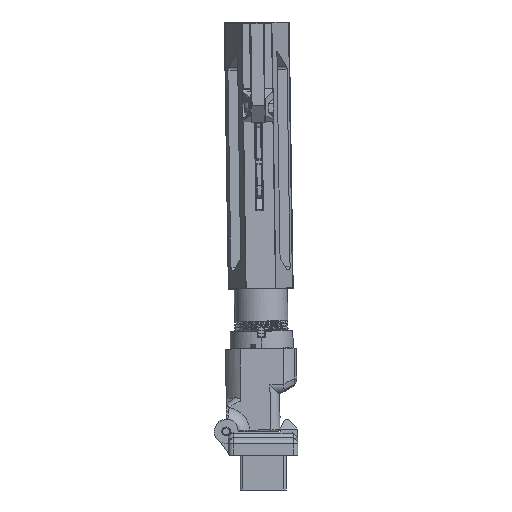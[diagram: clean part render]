
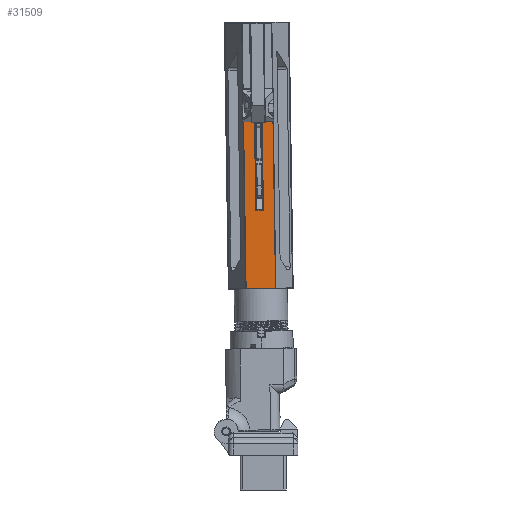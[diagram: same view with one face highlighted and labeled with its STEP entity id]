
A CAD part, front view. The second image highlights one B-rep face of the part: STEP entity #31509.
In plain terms, the highlighted planar face has unit normal (0.001, -1, 0).
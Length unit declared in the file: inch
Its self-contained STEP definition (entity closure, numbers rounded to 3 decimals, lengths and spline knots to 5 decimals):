
#1038 = DIRECTION ( 'NONE',  ( -1., 0., 0. ) ) ;
#1393 = EDGE_CURVE ( 'NONE', #83956, #16129, #110969, .T. ) ;
#1433 = LINE ( 'NONE', #73468, #92094 ) ;
#1583 = CARTESIAN_POINT ( 'NONE',  ( -0.20623, 2.27701, 0.60654 ) ) ;
#3004 = LINE ( 'NONE', #113807, #50618 ) ;
#4150 = CARTESIAN_POINT ( 'NONE',  ( 0.25882, 2.27701, 0.75605 ) ) ;
#4573 = EDGE_CURVE ( 'NONE', #48424, #16129, #3004, .T. ) ;
#5254 = VECTOR ( 'NONE', #115520, 39.37008 ) ;
#6679 = LINE ( 'NONE', #60556, #40078 ) ;
#7333 = VERTEX_POINT ( 'NONE', #119775 ) ;
#7878 = DIRECTION ( 'NONE',  ( -1., 0., 0. ) ) ;
#9898 = DIRECTION ( 'NONE',  ( 0., 0., 1. ) ) ;
#11533 = CARTESIAN_POINT ( 'NONE',  ( 0.25882, 2.27701, 4.21059 ) ) ;
#11699 = LINE ( 'NONE', #93976, #109061 ) ;
#12814 = VECTOR ( 'NONE', #1038, 39.37008 ) ;
#13151 = DIRECTION ( 'NONE',  ( 0., 0., -1. ) ) ;
#14095 = EDGE_CURVE ( 'NONE', #109037, #54313, #96042, .T. ) ;
#14333 = VERTEX_POINT ( 'NONE', #36059 ) ;
#14604 = EDGE_LOOP ( 'NONE', ( #80668, #86055, #26712, #99197, #62341, #112582, #38522, #43325, #58567, #66247, #104048, #114836 ) ) ;
#16129 = VERTEX_POINT ( 'NONE', #95921 ) ;
#17422 = VECTOR ( 'NONE', #95929, 39.37008 ) ;
#21709 = EDGE_CURVE ( 'NONE', #53142, #81474, #23504, .T. ) ;
#23504 = LINE ( 'NONE', #78538, #5254 ) ;
#26712 = ORIENTED_EDGE ( 'NONE', *, *, #64079, .T. ) ;
#28824 = VECTOR ( 'NONE', #64938, 39.37008 ) ;
#30843 = DIRECTION ( 'NONE',  ( 0., 0., -1. ) ) ;
#31509 = ADVANCED_FACE ( 'NONE', ( #77946 ), #68283, .T. ) ;
#32437 = LINE ( 'NONE', #69942, #37668 ) ;
#33949 = VECTOR ( 'NONE', #9898, 39.37008 ) ;
#34353 = CARTESIAN_POINT ( 'NONE',  ( 0.42972, 2.27701, 4.21059 ) ) ;
#36059 = CARTESIAN_POINT ( 'NONE',  ( 0.02853, 2.27701, 4.21414 ) ) ;
#37166 = AXIS2_PLACEMENT_3D ( 'NONE', #4150, #67688, #59822 ) ;
#37581 = VECTOR ( 'NONE', #13151, 39.37008 ) ;
#37668 = VECTOR ( 'NONE', #40341, 39.37008 ) ;
#38384 = DIRECTION ( 'NONE',  ( 0., 0., -1. ) ) ;
#38522 = ORIENTED_EDGE ( 'NONE', *, *, #71679, .T. ) ;
#40078 = VECTOR ( 'NONE', #7878, 39.37008 ) ;
#40341 = DIRECTION ( 'NONE',  ( -1., 0., 0. ) ) ;
#43325 = ORIENTED_EDGE ( 'NONE', *, *, #103541, .T. ) ;
#47232 = EDGE_CURVE ( 'NONE', #54313, #78135, #68656, .T. ) ;
#47954 = LINE ( 'NONE', #112142, #33949 ) ;
#48424 = VERTEX_POINT ( 'NONE', #67642 ) ;
#50618 = VECTOR ( 'NONE', #30843, 39.37008 ) ;
#53142 = VERTEX_POINT ( 'NONE', #85937 ) ;
#54313 = VERTEX_POINT ( 'NONE', #1583 ) ;
#58567 = ORIENTED_EDGE ( 'NONE', *, *, #105902, .T. ) ;
#59503 = CARTESIAN_POINT ( 'NONE',  ( -0.20623, 2.27701, 4.21059 ) ) ;
#59822 = DIRECTION ( 'NONE',  ( 0., 0., -1. ) ) ;
#60556 = CARTESIAN_POINT ( 'NONE',  ( 0.25882, 2.27701, 4.21414 ) ) ;
#61185 = VECTOR ( 'NONE', #65089, 39.37008 ) ;
#62341 = ORIENTED_EDGE ( 'NONE', *, *, #4573, .F. ) ;
#64079 = EDGE_CURVE ( 'NONE', #78135, #83956, #11699, .T. ) ;
#64938 = DIRECTION ( 'NONE',  ( -1., 0., 0. ) ) ;
#65089 = DIRECTION ( 'NONE',  ( -1., 0., 0. ) ) ;
#66247 = ORIENTED_EDGE ( 'NONE', *, *, #109834, .T. ) ;
#67489 = CARTESIAN_POINT ( 'NONE',  ( 0.42972, 2.27701, 0.60654 ) ) ;
#67642 = CARTESIAN_POINT ( 'NONE',  ( 0.25882, 2.27701, 4.21327 ) ) ;
#67688 = DIRECTION ( 'NONE',  ( 0., -1., 0. ) ) ;
#68283 = PLANE ( 'NONE',  #37166 ) ;
#68656 = LINE ( 'NONE', #77717, #17422 ) ;
#69942 = CARTESIAN_POINT ( 'NONE',  ( 0.25882, 2.27701, 2.2914 ) ) ;
#70063 = EDGE_CURVE ( 'NONE', #48424, #7333, #82619, .T. ) ;
#71679 = EDGE_CURVE ( 'NONE', #7333, #83482, #1433, .T. ) ;
#73468 = CARTESIAN_POINT ( 'NONE',  ( 0.19496, 2.27701, 0.75605 ) ) ;
#74956 = EDGE_CURVE ( 'NONE', #81474, #109037, #119142, .T. ) ;
#77717 = CARTESIAN_POINT ( 'NONE',  ( 0.42836, 2.27701, 0.60654 ) ) ;
#77946 = FACE_OUTER_BOUND ( 'NONE', #14604, .T. ) ;
#78135 = VERTEX_POINT ( 'NONE', #67489 ) ;
#78538 = CARTESIAN_POINT ( 'NONE',  ( -0.03533, 2.27701, 4.54102 ) ) ;
#80668 = ORIENTED_EDGE ( 'NONE', *, *, #14095, .T. ) ;
#81229 = CARTESIAN_POINT ( 'NONE',  ( -0.03533, 2.27701, 4.21059 ) ) ;
#81474 = VERTEX_POINT ( 'NONE', #81229 ) ;
#82619 = LINE ( 'NONE', #92325, #61185 ) ;
#83482 = VERTEX_POINT ( 'NONE', #107567 ) ;
#83933 = CARTESIAN_POINT ( 'NONE',  ( 0.25882, 2.27701, 4.21059 ) ) ;
#83956 = VERTEX_POINT ( 'NONE', #34353 ) ;
#85937 = CARTESIAN_POINT ( 'NONE',  ( -0.03533, 2.27701, 4.21414 ) ) ;
#86055 = ORIENTED_EDGE ( 'NONE', *, *, #47232, .T. ) ;
#86669 = DIRECTION ( 'NONE',  ( 0., 0., 1. ) ) ;
#87229 = VERTEX_POINT ( 'NONE', #103442 ) ;
#88125 = CARTESIAN_POINT ( 'NONE',  ( -0.20623, 2.27701, 0.75605 ) ) ;
#92094 = VECTOR ( 'NONE', #38384, 39.37008 ) ;
#92325 = CARTESIAN_POINT ( 'NONE',  ( 0.25882, 2.27701, 4.21327 ) ) ;
#93976 = CARTESIAN_POINT ( 'NONE',  ( 0.42972, 2.27701, 0.75605 ) ) ;
#95921 = CARTESIAN_POINT ( 'NONE',  ( 0.25882, 2.27701, 4.21059 ) ) ;
#95929 = DIRECTION ( 'NONE',  ( 1., 0., 0. ) ) ;
#96042 = LINE ( 'NONE', #88125, #37581 ) ;
#99197 = ORIENTED_EDGE ( 'NONE', *, *, #1393, .T. ) ;
#103442 = CARTESIAN_POINT ( 'NONE',  ( 0.02853, 2.27701, 2.2914 ) ) ;
#103541 = EDGE_CURVE ( 'NONE', #83482, #87229, #32437, .T. ) ;
#104048 = ORIENTED_EDGE ( 'NONE', *, *, #21709, .T. ) ;
#105902 = EDGE_CURVE ( 'NONE', #87229, #14333, #47954, .T. ) ;
#107567 = CARTESIAN_POINT ( 'NONE',  ( 0.19496, 2.27701, 2.2914 ) ) ;
#109037 = VERTEX_POINT ( 'NONE', #59503 ) ;
#109061 = VECTOR ( 'NONE', #86669, 39.37008 ) ;
#109834 = EDGE_CURVE ( 'NONE', #14333, #53142, #6679, .T. ) ;
#110969 = LINE ( 'NONE', #11533, #28824 ) ;
#112142 = CARTESIAN_POINT ( 'NONE',  ( 0.02853, 2.27701, 4.21414 ) ) ;
#112582 = ORIENTED_EDGE ( 'NONE', *, *, #70063, .T. ) ;
#113807 = CARTESIAN_POINT ( 'NONE',  ( 0.25882, 2.27701, 4.22027 ) ) ;
#114836 = ORIENTED_EDGE ( 'NONE', *, *, #74956, .T. ) ;
#115520 = DIRECTION ( 'NONE',  ( 0., 0., -1. ) ) ;
#119142 = LINE ( 'NONE', #83933, #12814 ) ;
#119775 = CARTESIAN_POINT ( 'NONE',  ( 0.19496, 2.27701, 4.21327 ) ) ;
